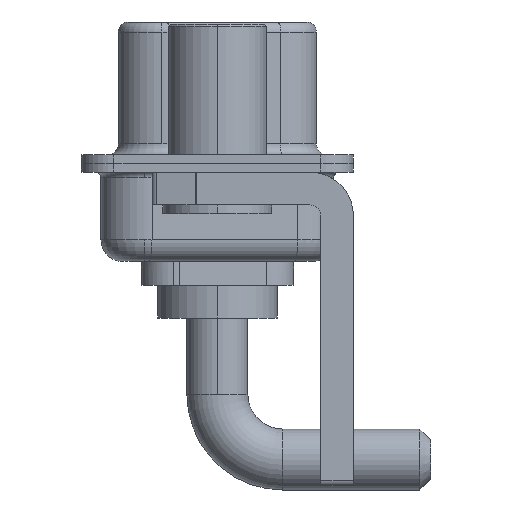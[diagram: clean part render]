
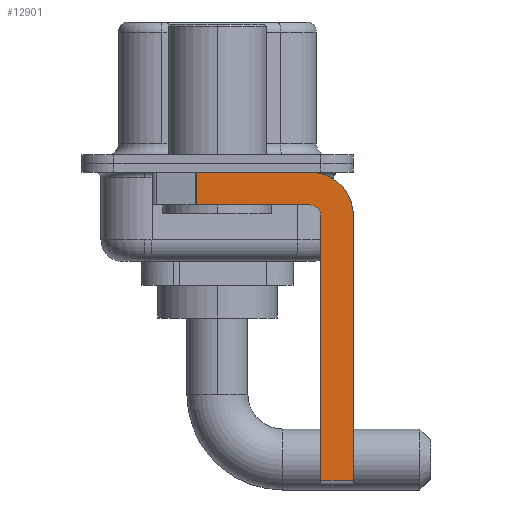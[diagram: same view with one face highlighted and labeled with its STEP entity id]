
A CAD part, left-side view. The second image highlights one B-rep face of the part: STEP entity #12901.
In plain terms, the highlighted planar face has unit normal (-1, 0, 0).
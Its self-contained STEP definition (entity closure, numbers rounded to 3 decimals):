
#158 = VECTOR ( 'NONE', #16278, 1000. ) ;
#347 = LINE ( 'NONE', #16584, #4657 ) ;
#685 = DIRECTION ( 'NONE',  ( 1., 0., 0. ) ) ;
#704 = CARTESIAN_POINT ( 'NONE',  ( -2.9, -4.25, -1.9 ) ) ;
#792 = CARTESIAN_POINT ( 'NONE',  ( -2.9, 0.978, -1.9 ) ) ;
#842 = CARTESIAN_POINT ( 'NONE',  ( -2.9, -4.25, -2.4 ) ) ;
#1063 = ORIENTED_EDGE ( 'NONE', *, *, #1098, .F. ) ;
#1098 = EDGE_CURVE ( 'NONE', #5333, #13400, #15083, .T. ) ;
#1547 = CARTESIAN_POINT ( 'NONE',  ( -2.9, -6.25, -2.4 ) ) ;
#1610 = VERTEX_POINT ( 'NONE', #1547 ) ;
#1613 = LINE ( 'NONE', #8377, #14755 ) ;
#2149 = CARTESIAN_POINT ( 'NONE',  ( -2.9, -6.25, -14.55 ) ) ;
#2460 = DIRECTION ( 'NONE',  ( 0., 0., -1. ) ) ;
#2733 = CARTESIAN_POINT ( 'NONE',  ( -2.9, -4.25, -2.4 ) ) ;
#3057 = VERTEX_POINT ( 'NONE', #4790 ) ;
#3130 = EDGE_CURVE ( 'NONE', #12624, #1610, #11287, .T. ) ;
#3549 = ORIENTED_EDGE ( 'NONE', *, *, #10469, .T. ) ;
#4103 = VECTOR ( 'NONE', #14026, 1000. ) ;
#4657 = VECTOR ( 'NONE', #6837, 1000. ) ;
#4790 = CARTESIAN_POINT ( 'NONE',  ( -2.9, 0.978, -0.4 ) ) ;
#5280 = CIRCLE ( 'NONE', #9929, 0.5 ) ;
#5333 = VERTEX_POINT ( 'NONE', #7202 ) ;
#5921 = LINE ( 'NONE', #792, #13418 ) ;
#6056 = LINE ( 'NONE', #10279, #12392 ) ;
#6064 = CARTESIAN_POINT ( 'NONE',  ( -2.9, -4.25, -2.4 ) ) ;
#6072 = ORIENTED_EDGE ( 'NONE', *, *, #10770, .T. ) ;
#6837 = DIRECTION ( 'NONE',  ( 0., 0., 1. ) ) ;
#6916 = ORIENTED_EDGE ( 'NONE', *, *, #7260, .F. ) ;
#7202 = CARTESIAN_POINT ( 'NONE',  ( -2.9, -4.25, -1.9 ) ) ;
#7260 = EDGE_CURVE ( 'NONE', #3057, #12624, #1613, .T. ) ;
#8377 = CARTESIAN_POINT ( 'NONE',  ( -2.9, 3., -0.4 ) ) ;
#8596 = CARTESIAN_POINT ( 'NONE',  ( -2.9, -4.75, -14.55 ) ) ;
#8640 = EDGE_CURVE ( 'NONE', #16432, #14392, #347, .T. ) ;
#8722 = FACE_OUTER_BOUND ( 'NONE', #9585, .T. ) ;
#8879 = CARTESIAN_POINT ( 'NONE',  ( -2.9, 0.978, -1.9 ) ) ;
#8999 = ORIENTED_EDGE ( 'NONE', *, *, #3130, .F. ) ;
#9201 = ORIENTED_EDGE ( 'NONE', *, *, #12591, .F. ) ;
#9585 = EDGE_LOOP ( 'NONE', ( #6916, #6072, #1063, #9201, #9644, #3549, #16055, #8999 ) ) ;
#9642 = AXIS2_PLACEMENT_3D ( 'NONE', #6064, #685, #12244 ) ;
#9644 = ORIENTED_EDGE ( 'NONE', *, *, #8640, .F. ) ;
#9929 = AXIS2_PLACEMENT_3D ( 'NONE', #2733, #14406, #14724 ) ;
#10007 = LINE ( 'NONE', #15487, #4103 ) ;
#10090 = PLANE ( 'NONE',  #10221 ) ;
#10221 = AXIS2_PLACEMENT_3D ( 'NONE', #842, #16854, #2460 ) ;
#10279 = CARTESIAN_POINT ( 'NONE',  ( -2.9, -6.25, -2.4 ) ) ;
#10469 = EDGE_CURVE ( 'NONE', #16432, #16844, #10007, .T. ) ;
#10770 = EDGE_CURVE ( 'NONE', #3057, #13400, #5921, .T. ) ;
#10905 = CARTESIAN_POINT ( 'NONE',  ( -2.9, -4.75, -2.4 ) ) ;
#11287 = CIRCLE ( 'NONE', #9642, 2. ) ;
#11302 = DIRECTION ( 'NONE',  ( 0., 0., -1. ) ) ;
#11917 = CARTESIAN_POINT ( 'NONE',  ( -2.9, -4.25, -0.4 ) ) ;
#12150 = DIRECTION ( 'NONE',  ( 0., -1., 0. ) ) ;
#12244 = DIRECTION ( 'NONE',  ( 0., 0., -1. ) ) ;
#12392 = VECTOR ( 'NONE', #11302, 1000. ) ;
#12591 = EDGE_CURVE ( 'NONE', #14392, #5333, #5280, .T. ) ;
#12624 = VERTEX_POINT ( 'NONE', #11917 ) ;
#12901 = ADVANCED_FACE ( 'NONE', ( #8722 ), #10090, .F. ) ;
#12927 = EDGE_CURVE ( 'NONE', #1610, #16844, #6056, .T. ) ;
#13400 = VERTEX_POINT ( 'NONE', #8879 ) ;
#13418 = VECTOR ( 'NONE', #13821, 1000. ) ;
#13821 = DIRECTION ( 'NONE',  ( 0., 0., -1. ) ) ;
#14026 = DIRECTION ( 'NONE',  ( 0., -1., 0. ) ) ;
#14392 = VERTEX_POINT ( 'NONE', #10905 ) ;
#14406 = DIRECTION ( 'NONE',  ( -1., 0., 0. ) ) ;
#14724 = DIRECTION ( 'NONE',  ( 0., 0., 1. ) ) ;
#14755 = VECTOR ( 'NONE', #12150, 1000. ) ;
#15083 = LINE ( 'NONE', #704, #158 ) ;
#15487 = CARTESIAN_POINT ( 'NONE',  ( -2.9, -4.25, -14.55 ) ) ;
#16055 = ORIENTED_EDGE ( 'NONE', *, *, #12927, .F. ) ;
#16278 = DIRECTION ( 'NONE',  ( 0., 1., 0. ) ) ;
#16432 = VERTEX_POINT ( 'NONE', #8596 ) ;
#16584 = CARTESIAN_POINT ( 'NONE',  ( -2.9, -4.75, -14.8 ) ) ;
#16844 = VERTEX_POINT ( 'NONE', #2149 ) ;
#16854 = DIRECTION ( 'NONE',  ( 1., 0., 0. ) ) ;
